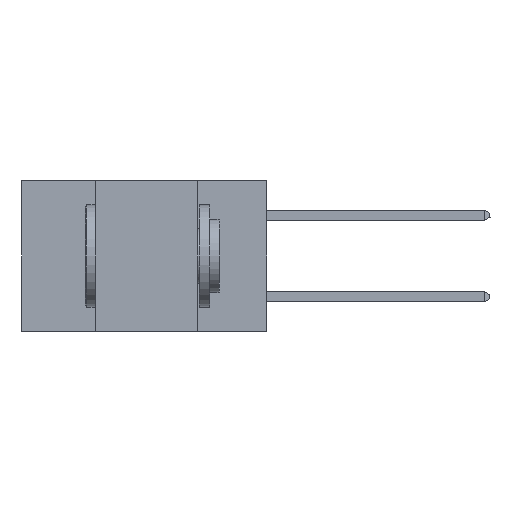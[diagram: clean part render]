
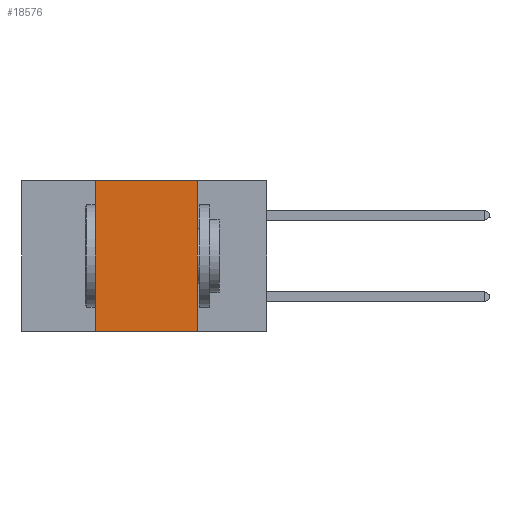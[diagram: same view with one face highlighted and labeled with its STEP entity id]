
A CAD part, left-side view. The second image highlights one B-rep face of the part: STEP entity #18576.
In plain terms, the highlighted planar face has unit normal (-1, 0, 0).
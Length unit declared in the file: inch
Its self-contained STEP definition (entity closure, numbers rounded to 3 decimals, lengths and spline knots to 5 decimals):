
#537 = DIRECTION ( 'NONE',  ( 0., 0., -1. ) ) ;
#723 = CARTESIAN_POINT ( 'NONE',  ( 0., 0.42, -0.37 ) ) ;
#740 = CARTESIAN_POINT ( 'NONE',  ( 0., 0.6, 0. ) ) ;
#786 = FACE_OUTER_BOUND ( 'NONE', #1916, .T. ) ;
#1142 = CARTESIAN_POINT ( 'NONE',  ( 0., 0.17, -0.37 ) ) ;
#1916 = EDGE_LOOP ( 'NONE', ( #10954, #25024, #16821, #18701 ) ) ;
#3342 = VECTOR ( 'NONE', #11304, 39.37008 ) ;
#3476 = LINE ( 'NONE', #12777, #16621 ) ;
#5057 = CARTESIAN_POINT ( 'NONE',  ( 0., 0.6, 0. ) ) ;
#5461 = VERTEX_POINT ( 'NONE', #723 ) ;
#6687 = PLANE ( 'NONE',  #22791 ) ;
#9040 = LINE ( 'NONE', #9671, #18430 ) ;
#9631 = VERTEX_POINT ( 'NONE', #1142 ) ;
#9671 = CARTESIAN_POINT ( 'NONE',  ( 0., 0.6, -0.37 ) ) ;
#10954 = ORIENTED_EDGE ( 'NONE', *, *, #14267, .F. ) ;
#11304 = DIRECTION ( 'NONE',  ( 0., -1., 0. ) ) ;
#12777 = CARTESIAN_POINT ( 'NONE',  ( 0., 0.17, 0. ) ) ;
#12991 = DIRECTION ( 'NONE',  ( 0., 0., -1. ) ) ;
#13578 = CARTESIAN_POINT ( 'NONE',  ( 0., 0.42, 0. ) ) ;
#14267 = EDGE_CURVE ( 'NONE', #21043, #9631, #3476, .T. ) ;
#15782 = DIRECTION ( 'NONE',  ( 0., -1., 0. ) ) ;
#16305 = EDGE_CURVE ( 'NONE', #5461, #9631, #9040, .T. ) ;
#16621 = VECTOR ( 'NONE', #537, 39.37008 ) ;
#16821 = ORIENTED_EDGE ( 'NONE', *, *, #20662, .F. ) ;
#17466 = VERTEX_POINT ( 'NONE', #17889 ) ;
#17585 = DIRECTION ( 'NONE',  ( 0., 0., 1. ) ) ;
#17889 = CARTESIAN_POINT ( 'NONE',  ( 0., 0.42, 0. ) ) ;
#17995 = LINE ( 'NONE', #13578, #23980 ) ;
#18430 = VECTOR ( 'NONE', #15782, 39.37008 ) ;
#18576 = ADVANCED_FACE ( 'NONE', ( #786 ), #6687, .F. ) ;
#18701 = ORIENTED_EDGE ( 'NONE', *, *, #16305, .T. ) ;
#20662 = EDGE_CURVE ( 'NONE', #5461, #17466, #17995, .T. ) ;
#21043 = VERTEX_POINT ( 'NONE', #23114 ) ;
#21569 = LINE ( 'NONE', #5057, #3342 ) ;
#22791 = AXIS2_PLACEMENT_3D ( 'NONE', #740, #25019, #12991 ) ;
#23114 = CARTESIAN_POINT ( 'NONE',  ( 0., 0.17, 0. ) ) ;
#23980 = VECTOR ( 'NONE', #17585, 39.37008 ) ;
#25019 = DIRECTION ( 'NONE',  ( 1., 0., 0. ) ) ;
#25024 = ORIENTED_EDGE ( 'NONE', *, *, #25625, .F. ) ;
#25625 = EDGE_CURVE ( 'NONE', #17466, #21043, #21569, .T. ) ;
